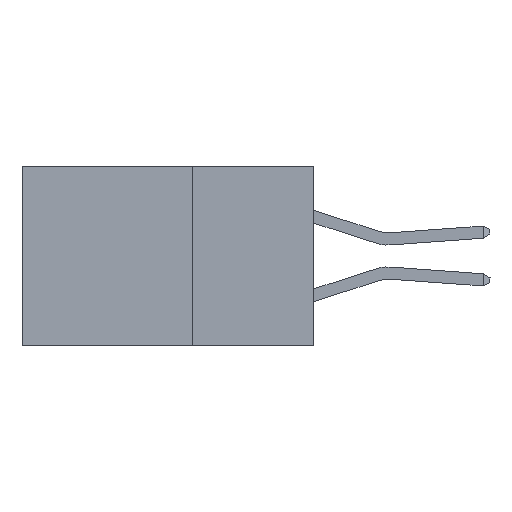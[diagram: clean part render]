
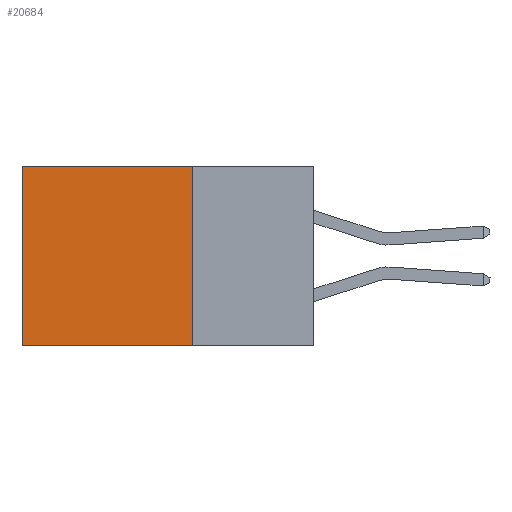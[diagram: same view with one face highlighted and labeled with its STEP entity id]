
A CAD part, left-side view. The second image highlights one B-rep face of the part: STEP entity #20684.
In plain terms, the highlighted planar face has unit normal (-1, 0, 0).
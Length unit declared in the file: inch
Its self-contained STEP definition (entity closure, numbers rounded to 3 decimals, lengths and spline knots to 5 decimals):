
#521 = CARTESIAN_POINT ( 'NONE',  ( 0.2875, 0.25, -0.37 ) ) ;
#2672 = VECTOR ( 'NONE', #20240, 39.37008 ) ;
#3598 = CARTESIAN_POINT ( 'NONE',  ( 0.2875, 0.6, 0. ) ) ;
#3600 = LINE ( 'NONE', #9012, #14530 ) ;
#4474 = EDGE_CURVE ( 'NONE', #27061, #11807, #8672, .T. ) ;
#4762 = VECTOR ( 'NONE', #34289, 39.37008 ) ;
#5646 = EDGE_CURVE ( 'NONE', #35201, #31342, #28697, .T. ) ;
#6375 = DIRECTION ( 'NONE',  ( 0., 1., 0. ) ) ;
#7183 = CARTESIAN_POINT ( 'NONE',  ( 0.2875, 0.25, 0. ) ) ;
#7492 = EDGE_LOOP ( 'NONE', ( #14430, #26731, #17737, #28851 ) ) ;
#8672 = LINE ( 'NONE', #34839, #2672 ) ;
#9012 = CARTESIAN_POINT ( 'NONE',  ( 0.2875, 0.25, -0.37 ) ) ;
#9677 = DIRECTION ( 'NONE',  ( 1., 0., 0. ) ) ;
#11807 = VERTEX_POINT ( 'NONE', #37464 ) ;
#14430 = ORIENTED_EDGE ( 'NONE', *, *, #4474, .T. ) ;
#14530 = VECTOR ( 'NONE', #15179, 39.37008 ) ;
#15179 = DIRECTION ( 'NONE',  ( 0., 1., 0. ) ) ;
#17737 = ORIENTED_EDGE ( 'NONE', *, *, #5646, .F. ) ;
#18370 = DIRECTION ( 'NONE',  ( 0., 0., -1. ) ) ;
#20240 = DIRECTION ( 'NONE',  ( 0., 0., -1. ) ) ;
#20684 = ADVANCED_FACE ( 'NONE', ( #21435 ), #36439, .F. ) ;
#21008 = LINE ( 'NONE', #24279, #22696 ) ;
#21435 = FACE_OUTER_BOUND ( 'NONE', #7492, .T. ) ;
#21525 = EDGE_CURVE ( 'NONE', #31342, #11807, #3600, .T. ) ;
#22218 = CARTESIAN_POINT ( 'NONE',  ( 0.2875, 0.25, 0. ) ) ;
#22696 = VECTOR ( 'NONE', #6375, 39.37008 ) ;
#24279 = CARTESIAN_POINT ( 'NONE',  ( 0.2875, 0.25, 0. ) ) ;
#25817 = CARTESIAN_POINT ( 'NONE',  ( 0.2875, 0.25, 0. ) ) ;
#26731 = ORIENTED_EDGE ( 'NONE', *, *, #21525, .F. ) ;
#27061 = VERTEX_POINT ( 'NONE', #3598 ) ;
#28697 = LINE ( 'NONE', #25817, #4762 ) ;
#28851 = ORIENTED_EDGE ( 'NONE', *, *, #32174, .T. ) ;
#30507 = AXIS2_PLACEMENT_3D ( 'NONE', #7183, #9677, #18370 ) ;
#31342 = VERTEX_POINT ( 'NONE', #521 ) ;
#32174 = EDGE_CURVE ( 'NONE', #35201, #27061, #21008, .T. ) ;
#34289 = DIRECTION ( 'NONE',  ( 0., 0., -1. ) ) ;
#34839 = CARTESIAN_POINT ( 'NONE',  ( 0.2875, 0.6, 0. ) ) ;
#35201 = VERTEX_POINT ( 'NONE', #22218 ) ;
#36439 = PLANE ( 'NONE',  #30507 ) ;
#37464 = CARTESIAN_POINT ( 'NONE',  ( 0.2875, 0.6, -0.37 ) ) ;
